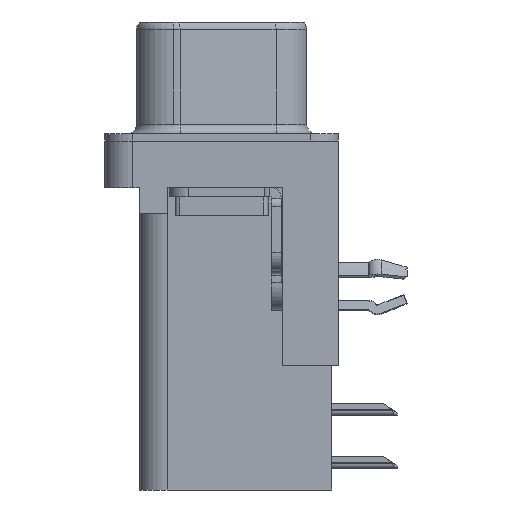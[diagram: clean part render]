
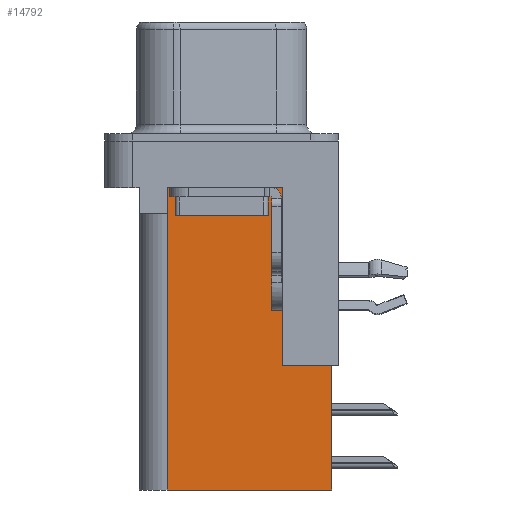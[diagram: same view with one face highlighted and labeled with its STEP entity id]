
A CAD part, left-side view. The second image highlights one B-rep face of the part: STEP entity #14792.
In plain terms, the highlighted planar face has unit normal (-1, 0, 0).
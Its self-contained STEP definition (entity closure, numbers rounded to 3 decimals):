
#436 = CARTESIAN_POINT ( 'NONE',  ( 3.79, 2.925, -18.76 ) ) ;
#579 = DIRECTION ( 'NONE',  ( 0., 0., 1. ) ) ;
#1145 = DIRECTION ( 'NONE',  ( 0., 0., -1. ) ) ;
#1312 = ORIENTED_EDGE ( 'NONE', *, *, #25489, .T. ) ;
#2123 = VECTOR ( 'NONE', #13237, 1000. ) ;
#2288 = LINE ( 'NONE', #22011, #2123 ) ;
#2401 = CARTESIAN_POINT ( 'NONE',  ( 3.79, -3.295, -18.76 ) ) ;
#2843 = FACE_OUTER_BOUND ( 'NONE', #20022, .T. ) ;
#2978 = VERTEX_POINT ( 'NONE', #17917 ) ;
#3267 = EDGE_CURVE ( 'NONE', #4685, #8714, #7234, .T. ) ;
#3403 = ORIENTED_EDGE ( 'NONE', *, *, #19429, .T. ) ;
#3769 = VERTEX_POINT ( 'NONE', #11087 ) ;
#4685 = VERTEX_POINT ( 'NONE', #18790 ) ;
#4777 = DIRECTION ( 'NONE',  ( 1., 0., 0. ) ) ;
#4892 = VERTEX_POINT ( 'NONE', #13094 ) ;
#5292 = EDGE_CURVE ( 'NONE', #28266, #8714, #18137, .T. ) ;
#5525 = CARTESIAN_POINT ( 'NONE',  ( 3.79, 2.895, -2.5 ) ) ;
#5640 = ORIENTED_EDGE ( 'NONE', *, *, #3267, .F. ) ;
#5842 = ORIENTED_EDGE ( 'NONE', *, *, #5292, .T. ) ;
#6047 = CARTESIAN_POINT ( 'NONE',  ( 3.79, -5.925, -18.76 ) ) ;
#7140 = VECTOR ( 'NONE', #579, 1000. ) ;
#7234 = LINE ( 'NONE', #436, #7140 ) ;
#8025 = VERTEX_POINT ( 'NONE', #5525 ) ;
#8714 = VERTEX_POINT ( 'NONE', #26619 ) ;
#10063 = CARTESIAN_POINT ( 'NONE',  ( 3.79, 2.895, -3.9 ) ) ;
#11087 = CARTESIAN_POINT ( 'NONE',  ( 3.79, -5.925, -12.05 ) ) ;
#12355 = VECTOR ( 'NONE', #20921, 1000. ) ;
#12464 = LINE ( 'NONE', #22927, #12355 ) ;
#13094 = CARTESIAN_POINT ( 'NONE',  ( 3.79, -3.295, -2.5 ) ) ;
#13237 = DIRECTION ( 'NONE',  ( 0., 1., 0. ) ) ;
#14004 = ORIENTED_EDGE ( 'NONE', *, *, #21855, .T. ) ;
#14568 = CARTESIAN_POINT ( 'NONE',  ( 3.79, 2.895, -3.9 ) ) ;
#14792 = ADVANCED_FACE ( 'NONE', ( #2843 ), #16189, .F. ) ;
#15205 = DIRECTION ( 'NONE',  ( 0., 1., 0. ) ) ;
#16189 = PLANE ( 'NONE',  #26507 ) ;
#16796 = DIRECTION ( 'NONE',  ( 0., 0., -1. ) ) ;
#16952 = ORIENTED_EDGE ( 'NONE', *, *, #24182, .F. ) ;
#17189 = VECTOR ( 'NONE', #16796, 1000. ) ;
#17277 = LINE ( 'NONE', #14568, #17189 ) ;
#17446 = VECTOR ( 'NONE', #23768, 1000. ) ;
#17477 = LINE ( 'NONE', #21864, #17446 ) ;
#17917 = CARTESIAN_POINT ( 'NONE',  ( 3.79, -3.295, -12.05 ) ) ;
#18085 = VECTOR ( 'NONE', #25409, 1000. ) ;
#18137 = LINE ( 'NONE', #27530, #18085 ) ;
#18790 = CARTESIAN_POINT ( 'NONE',  ( 3.79, 2.925, -18.76 ) ) ;
#18997 = VERTEX_POINT ( 'NONE', #6047 ) ;
#19022 = EDGE_CURVE ( 'NONE', #4892, #8025, #17477, .T. ) ;
#19429 = EDGE_CURVE ( 'NONE', #2978, #4892, #12464, .T. ) ;
#19727 = ORIENTED_EDGE ( 'NONE', *, *, #22494, .F. ) ;
#20022 = EDGE_LOOP ( 'NONE', ( #25426, #1312, #5842, #5640, #16952, #19727, #14004, #3403 ) ) ;
#20654 = DIRECTION ( 'NONE',  ( 0., 1., 0. ) ) ;
#20921 = DIRECTION ( 'NONE',  ( 0., 0., 1. ) ) ;
#21855 = EDGE_CURVE ( 'NONE', #3769, #2978, #2288, .T. ) ;
#21864 = CARTESIAN_POINT ( 'NONE',  ( 3.79, -3.295, -2.5 ) ) ;
#22011 = CARTESIAN_POINT ( 'NONE',  ( 3.79, -6.295, -12.05 ) ) ;
#22297 = VECTOR ( 'NONE', #15205, 1000. ) ;
#22494 = EDGE_CURVE ( 'NONE', #3769, #18997, #27829, .T. ) ;
#22547 = LINE ( 'NONE', #28036, #22297 ) ;
#22927 = CARTESIAN_POINT ( 'NONE',  ( 3.79, -3.295, -18.76 ) ) ;
#23694 = CARTESIAN_POINT ( 'NONE',  ( 3.79, -5.925, -2. ) ) ;
#23768 = DIRECTION ( 'NONE',  ( 0., 1., 0. ) ) ;
#24182 = EDGE_CURVE ( 'NONE', #18997, #4685, #22547, .T. ) ;
#25409 = DIRECTION ( 'NONE',  ( 0., 1., 0. ) ) ;
#25426 = ORIENTED_EDGE ( 'NONE', *, *, #19022, .T. ) ;
#25489 = EDGE_CURVE ( 'NONE', #8025, #28266, #17277, .T. ) ;
#26507 = AXIS2_PLACEMENT_3D ( 'NONE', #2401, #4777, #20654 ) ;
#26619 = CARTESIAN_POINT ( 'NONE',  ( 3.79, 2.925, -3.9 ) ) ;
#27530 = CARTESIAN_POINT ( 'NONE',  ( 3.79, 0., -3.9 ) ) ;
#27803 = VECTOR ( 'NONE', #1145, 1000. ) ;
#27829 = LINE ( 'NONE', #23694, #27803 ) ;
#28036 = CARTESIAN_POINT ( 'NONE',  ( 3.79, -3.295, -18.76 ) ) ;
#28266 = VERTEX_POINT ( 'NONE', #10063 ) ;
